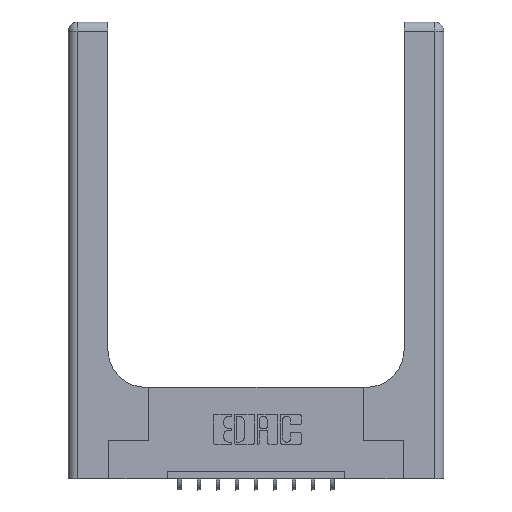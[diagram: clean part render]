
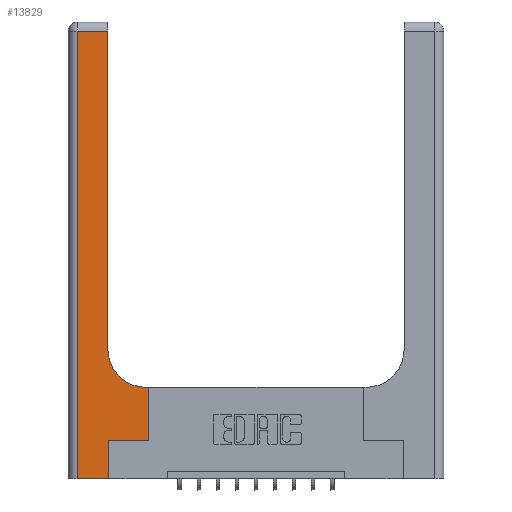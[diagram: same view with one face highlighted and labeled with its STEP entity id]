
A CAD part, top view. The second image highlights one B-rep face of the part: STEP entity #13829.
In plain terms, the highlighted planar face has unit normal (0, 0, 1).
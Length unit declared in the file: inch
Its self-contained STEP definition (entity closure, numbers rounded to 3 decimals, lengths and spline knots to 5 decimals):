
#40 = CARTESIAN_POINT ( 'NONE',  ( 0.51, 0.85, 0.37 ) ) ;
#94 = VECTOR ( 'NONE', #3439, 39.37008 ) ;
#447 = VERTEX_POINT ( 'NONE', #6881 ) ;
#605 = VERTEX_POINT ( 'NONE', #4375 ) ;
#908 = CARTESIAN_POINT ( 'NONE',  ( 0.265, 0.25, 0.37 ) ) ;
#1267 = CARTESIAN_POINT ( 'NONE',  ( 0.528, 0.25, 0.37 ) ) ;
#1289 = DIRECTION ( 'NONE',  ( 1., 0., 0. ) ) ;
#1525 = EDGE_CURVE ( 'NONE', #6485, #11449, #9922, .T. ) ;
#2429 = LINE ( 'NONE', #2773, #14559 ) ;
#2773 = CARTESIAN_POINT ( 'NONE',  ( 0.06, 3., 0.37 ) ) ;
#3014 = VECTOR ( 'NONE', #13265, 39.37008 ) ;
#3296 = EDGE_CURVE ( 'NONE', #8613, #12995, #13506, .T. ) ;
#3439 = DIRECTION ( 'NONE',  ( 0., 1., 0. ) ) ;
#3512 = VERTEX_POINT ( 'NONE', #9993 ) ;
#4115 = LINE ( 'NONE', #908, #7253 ) ;
#4137 = VECTOR ( 'NONE', #4897, 39.37008 ) ;
#4375 = CARTESIAN_POINT ( 'NONE',  ( 0.26, 2.94, 0.37 ) ) ;
#4674 = EDGE_CURVE ( 'NONE', #3512, #6485, #2429, .T. ) ;
#4705 = ORIENTED_EDGE ( 'NONE', *, *, #13940, .T. ) ;
#4710 = EDGE_LOOP ( 'NONE', ( #5578, #11628, #14599, #6800, #4705, #4837, #11044, #12108, #11993 ) ) ;
#4837 = ORIENTED_EDGE ( 'NONE', *, *, #14775, .T. ) ;
#4897 = DIRECTION ( 'NONE',  ( 0., 1., 0. ) ) ;
#5557 = VECTOR ( 'NONE', #11056, 39.37008 ) ;
#5578 = ORIENTED_EDGE ( 'NONE', *, *, #12912, .T. ) ;
#5831 = CARTESIAN_POINT ( 'NONE',  ( 0.26, 3., 0.37 ) ) ;
#6167 = DIRECTION ( 'NONE',  ( -1., 0., 0. ) ) ;
#6485 = VERTEX_POINT ( 'NONE', #10070 ) ;
#6800 = ORIENTED_EDGE ( 'NONE', *, *, #1525, .T. ) ;
#6877 = DIRECTION ( 'NONE',  ( 1., 0., 0. ) ) ;
#6881 = CARTESIAN_POINT ( 'NONE',  ( 0.26, 0.85, 0.37 ) ) ;
#7049 = EDGE_CURVE ( 'NONE', #10279, #447, #8298, .T. ) ;
#7149 = VECTOR ( 'NONE', #14167, 39.37008 ) ;
#7181 = VECTOR ( 'NONE', #8401, 39.37008 ) ;
#7249 = VERTEX_POINT ( 'NONE', #14923 ) ;
#7253 = VECTOR ( 'NONE', #6877, 39.37008 ) ;
#7375 = CARTESIAN_POINT ( 'NONE',  ( 0., 2.94, 0.37 ) ) ;
#7684 = AXIS2_PLACEMENT_3D ( 'NONE', #11982, #13174, #6167 ) ;
#8165 = EDGE_CURVE ( 'NONE', #12995, #10279, #10689, .T. ) ;
#8298 = CIRCLE ( 'NONE', #9687, 0.25 ) ;
#8325 = CARTESIAN_POINT ( 'NONE',  ( 0.528, 0.6, 0.37 ) ) ;
#8363 = CARTESIAN_POINT ( 'NONE',  ( 0., 0., 0.37 ) ) ;
#8401 = DIRECTION ( 'NONE',  ( -1., 0., 0. ) ) ;
#8433 = DIRECTION ( 'NONE',  ( 0., 0., -1. ) ) ;
#8595 = CARTESIAN_POINT ( 'NONE',  ( 0.51, 0.6, 0.37 ) ) ;
#8613 = VERTEX_POINT ( 'NONE', #9310 ) ;
#8695 = CARTESIAN_POINT ( 'NONE',  ( 0.265, 0., 0.37 ) ) ;
#9310 = CARTESIAN_POINT ( 'NONE',  ( 0.528, 0.25, 0.37 ) ) ;
#9687 = AXIS2_PLACEMENT_3D ( 'NONE', #40, #8433, #1289 ) ;
#9922 = LINE ( 'NONE', #8363, #7149 ) ;
#9993 = CARTESIAN_POINT ( 'NONE',  ( 0.06, 2.94, 0.37 ) ) ;
#10070 = CARTESIAN_POINT ( 'NONE',  ( 0.06, 0., 0.37 ) ) ;
#10185 = FACE_OUTER_BOUND ( 'NONE', #4710, .T. ) ;
#10279 = VERTEX_POINT ( 'NONE', #8595 ) ;
#10689 = LINE ( 'NONE', #11881, #7181 ) ;
#10860 = PLANE ( 'NONE',  #7684 ) ;
#11044 = ORIENTED_EDGE ( 'NONE', *, *, #3296, .T. ) ;
#11056 = DIRECTION ( 'NONE',  ( 0., 1., 0. ) ) ;
#11449 = VERTEX_POINT ( 'NONE', #13136 ) ;
#11628 = ORIENTED_EDGE ( 'NONE', *, *, #14375, .T. ) ;
#11881 = CARTESIAN_POINT ( 'NONE',  ( 0.26, 0.6, 0.37 ) ) ;
#11982 = CARTESIAN_POINT ( 'NONE',  ( 0., 3., 0.37 ) ) ;
#11993 = ORIENTED_EDGE ( 'NONE', *, *, #7049, .T. ) ;
#12108 = ORIENTED_EDGE ( 'NONE', *, *, #8165, .T. ) ;
#12193 = LINE ( 'NONE', #8695, #5557 ) ;
#12267 = DIRECTION ( 'NONE',  ( 0., -1., 0. ) ) ;
#12375 = LINE ( 'NONE', #5831, #94 ) ;
#12912 = EDGE_CURVE ( 'NONE', #447, #605, #12375, .T. ) ;
#12995 = VERTEX_POINT ( 'NONE', #8325 ) ;
#13136 = CARTESIAN_POINT ( 'NONE',  ( 0.265, 0., 0.37 ) ) ;
#13174 = DIRECTION ( 'NONE',  ( 0., 0., -1. ) ) ;
#13265 = DIRECTION ( 'NONE',  ( -1., 0., 0. ) ) ;
#13506 = LINE ( 'NONE', #1267, #4137 ) ;
#13829 = ADVANCED_FACE ( 'NONE', ( #10185 ), #10860, .F. ) ;
#13940 = EDGE_CURVE ( 'NONE', #11449, #7249, #12193, .T. ) ;
#14167 = DIRECTION ( 'NONE',  ( 1., 0., 0. ) ) ;
#14375 = EDGE_CURVE ( 'NONE', #605, #3512, #15108, .T. ) ;
#14559 = VECTOR ( 'NONE', #12267, 39.37008 ) ;
#14599 = ORIENTED_EDGE ( 'NONE', *, *, #4674, .T. ) ;
#14775 = EDGE_CURVE ( 'NONE', #7249, #8613, #4115, .T. ) ;
#14923 = CARTESIAN_POINT ( 'NONE',  ( 0.265, 0.25, 0.37 ) ) ;
#15108 = LINE ( 'NONE', #7375, #3014 ) ;
